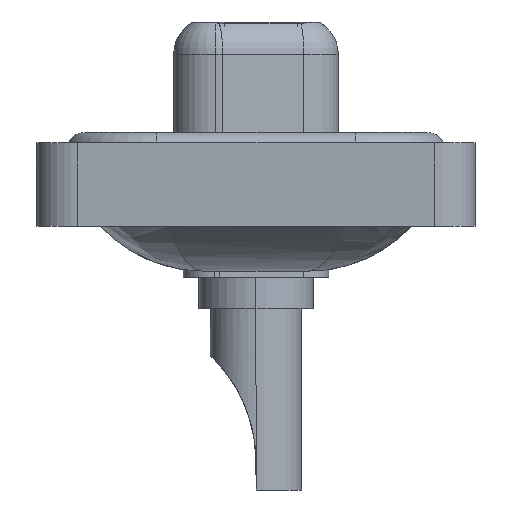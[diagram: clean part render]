
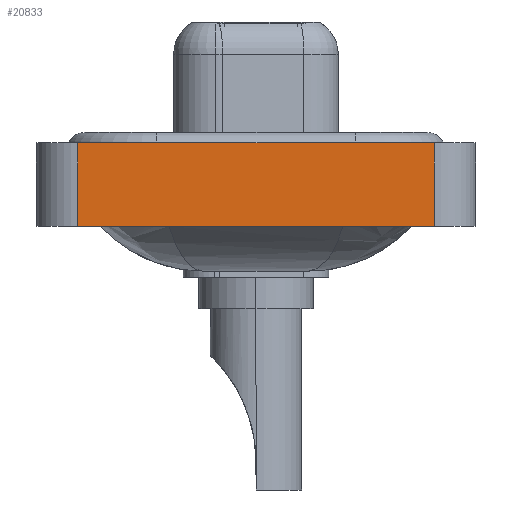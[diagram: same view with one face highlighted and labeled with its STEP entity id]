
A CAD part, left-side view. The second image highlights one B-rep face of the part: STEP entity #20833.
In plain terms, the highlighted planar face has unit normal (-1, 0, 0).
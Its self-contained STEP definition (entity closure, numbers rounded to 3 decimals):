
#53 = CARTESIAN_POINT ( 'NONE',  ( -7.35, 8.55, -3.6 ) ) ;
#66 = CARTESIAN_POINT ( 'NONE',  ( -7.35, -8.55, -3.6 ) ) ;
#479 = VECTOR ( 'NONE', #11586, 1000. ) ;
#706 = CARTESIAN_POINT ( 'NONE',  ( -7.35, -8.55, -3.6 ) ) ;
#800 = ORIENTED_EDGE ( 'NONE', *, *, #3704, .T. ) ;
#1355 = CARTESIAN_POINT ( 'NONE',  ( -7.35, -8.55, 0.4 ) ) ;
#2459 = EDGE_CURVE ( 'NONE', #19038, #13787, #8804, .T. ) ;
#2841 = DIRECTION ( 'NONE',  ( 0., 0., 1. ) ) ;
#3704 = EDGE_CURVE ( 'NONE', #19114, #19038, #13265, .T. ) ;
#3785 = AXIS2_PLACEMENT_3D ( 'NONE', #4451, #7750, #2841 ) ;
#4181 = CARTESIAN_POINT ( 'NONE',  ( -7.35, -8.55, 0.4 ) ) ;
#4451 = CARTESIAN_POINT ( 'NONE',  ( -7.35, -8.55, -3.6 ) ) ;
#6337 = CARTESIAN_POINT ( 'NONE',  ( -7.35, -8.55, -3.6 ) ) ;
#6626 = CARTESIAN_POINT ( 'NONE',  ( -7.35, 8.55, 0.4 ) ) ;
#6672 = LINE ( 'NONE', #19676, #479 ) ;
#7642 = LINE ( 'NONE', #1355, #10265 ) ;
#7750 = DIRECTION ( 'NONE',  ( -1., 0., 0. ) ) ;
#8804 = LINE ( 'NONE', #706, #17051 ) ;
#9137 = DIRECTION ( 'NONE',  ( 0., -1., 0. ) ) ;
#10265 = VECTOR ( 'NONE', #9137, 1000. ) ;
#10854 = FACE_OUTER_BOUND ( 'NONE', #19193, .T. ) ;
#11366 = DIRECTION ( 'NONE',  ( 0., -1., 0. ) ) ;
#11586 = DIRECTION ( 'NONE',  ( 0., 0., 1. ) ) ;
#12104 = ORIENTED_EDGE ( 'NONE', *, *, #20729, .F. ) ;
#13121 = EDGE_CURVE ( 'NONE', #19114, #13903, #6672, .T. ) ;
#13124 = ORIENTED_EDGE ( 'NONE', *, *, #2459, .T. ) ;
#13265 = LINE ( 'NONE', #66, #20748 ) ;
#13787 = VERTEX_POINT ( 'NONE', #4181 ) ;
#13903 = VERTEX_POINT ( 'NONE', #6626 ) ;
#17051 = VECTOR ( 'NONE', #20211, 1000. ) ;
#17349 = PLANE ( 'NONE',  #3785 ) ;
#19038 = VERTEX_POINT ( 'NONE', #6337 ) ;
#19114 = VERTEX_POINT ( 'NONE', #53 ) ;
#19193 = EDGE_LOOP ( 'NONE', ( #13124, #12104, #20873, #800 ) ) ;
#19676 = CARTESIAN_POINT ( 'NONE',  ( -7.35, 8.55, -3.6 ) ) ;
#20211 = DIRECTION ( 'NONE',  ( 0., 0., 1. ) ) ;
#20729 = EDGE_CURVE ( 'NONE', #13903, #13787, #7642, .T. ) ;
#20748 = VECTOR ( 'NONE', #11366, 1000. ) ;
#20833 = ADVANCED_FACE ( 'NONE', ( #10854 ), #17349, .T. ) ;
#20873 = ORIENTED_EDGE ( 'NONE', *, *, #13121, .F. ) ;
